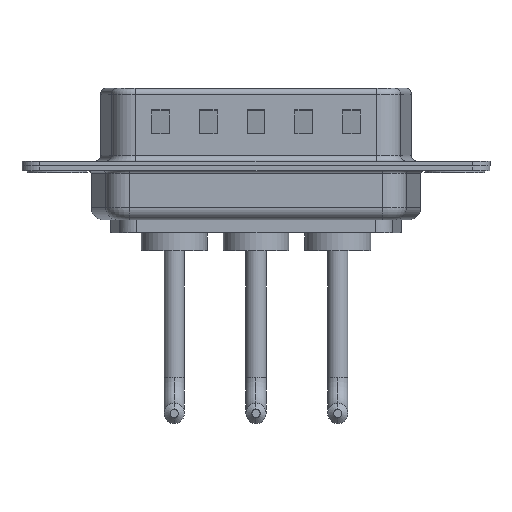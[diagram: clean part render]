
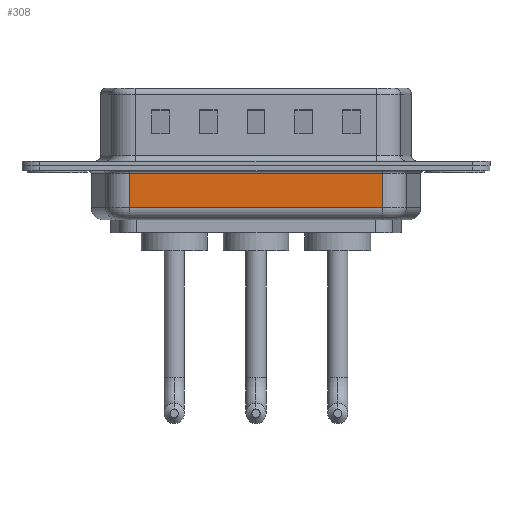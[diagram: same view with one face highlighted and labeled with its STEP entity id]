
A CAD part, front view. The second image highlights one B-rep face of the part: STEP entity #308.
In plain terms, the highlighted planar face has unit normal (0, -1, 0).
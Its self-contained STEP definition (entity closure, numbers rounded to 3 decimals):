
#239 = ORIENTED_EDGE ( 'NONE', *, *, #9900, .T. ) ;
#308 = ADVANCED_FACE ( 'NONE', ( #1691 ), #3868, .F. ) ;
#550 = VECTOR ( 'NONE', #7446, 1000. ) ;
#1182 = LINE ( 'NONE', #8546, #12825 ) ;
#1427 = VERTEX_POINT ( 'NONE', #6759 ) ;
#1691 = FACE_OUTER_BOUND ( 'NONE', #2209, .T. ) ;
#2209 = EDGE_LOOP ( 'NONE', ( #5964, #3004, #3852, #239 ) ) ;
#3004 = ORIENTED_EDGE ( 'NONE', *, *, #13698, .T. ) ;
#3380 = LINE ( 'NONE', #5407, #550 ) ;
#3568 = CARTESIAN_POINT ( 'NONE',  ( 27.269, -5.35, -3.5 ) ) ;
#3852 = ORIENTED_EDGE ( 'NONE', *, *, #8696, .T. ) ;
#3868 = PLANE ( 'NONE',  #8440 ) ;
#4552 = VERTEX_POINT ( 'NONE', #3568 ) ;
#5257 = CARTESIAN_POINT ( 'NONE',  ( 27.269, -5.35, -4.5 ) ) ;
#5407 = CARTESIAN_POINT ( 'NONE',  ( 6.031, -5.35, -3.5 ) ) ;
#5964 = ORIENTED_EDGE ( 'NONE', *, *, #8767, .F. ) ;
#6366 = DIRECTION ( 'NONE',  ( 0., 0., 1. ) ) ;
#6759 = CARTESIAN_POINT ( 'NONE',  ( 6.031, -5.35, -0.65 ) ) ;
#7352 = DIRECTION ( 'NONE',  ( 0., 0., 1. ) ) ;
#7446 = DIRECTION ( 'NONE',  ( 1., 0., 0. ) ) ;
#7988 = CARTESIAN_POINT ( 'NONE',  ( 27.269, -5.35, -0.65 ) ) ;
#8285 = DIRECTION ( 'NONE',  ( 0., 1., 0. ) ) ;
#8440 = AXIS2_PLACEMENT_3D ( 'NONE', #10328, #8285, #13555 ) ;
#8546 = CARTESIAN_POINT ( 'NONE',  ( 6.031, -5.35, -0.65 ) ) ;
#8662 = VERTEX_POINT ( 'NONE', #7988 ) ;
#8696 = EDGE_CURVE ( 'NONE', #4552, #8662, #11590, .T. ) ;
#8767 = EDGE_CURVE ( 'NONE', #10960, #1427, #11726, .T. ) ;
#9618 = CARTESIAN_POINT ( 'NONE',  ( 6.031, -5.35, -4.5 ) ) ;
#9888 = VECTOR ( 'NONE', #6366, 1000. ) ;
#9900 = EDGE_CURVE ( 'NONE', #8662, #1427, #1182, .T. ) ;
#10328 = CARTESIAN_POINT ( 'NONE',  ( 6.031, -5.35, -4.5 ) ) ;
#10960 = VERTEX_POINT ( 'NONE', #12875 ) ;
#11590 = LINE ( 'NONE', #5257, #13469 ) ;
#11726 = LINE ( 'NONE', #9618, #9888 ) ;
#12825 = VECTOR ( 'NONE', #13821, 1000. ) ;
#12875 = CARTESIAN_POINT ( 'NONE',  ( 6.031, -5.35, -3.5 ) ) ;
#13469 = VECTOR ( 'NONE', #7352, 1000. ) ;
#13555 = DIRECTION ( 'NONE',  ( 0., 0., 1. ) ) ;
#13698 = EDGE_CURVE ( 'NONE', #10960, #4552, #3380, .T. ) ;
#13821 = DIRECTION ( 'NONE',  ( -1., 0., 0. ) ) ;
